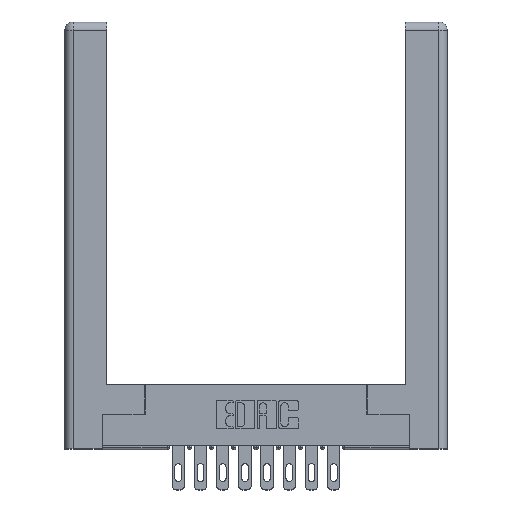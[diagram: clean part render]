
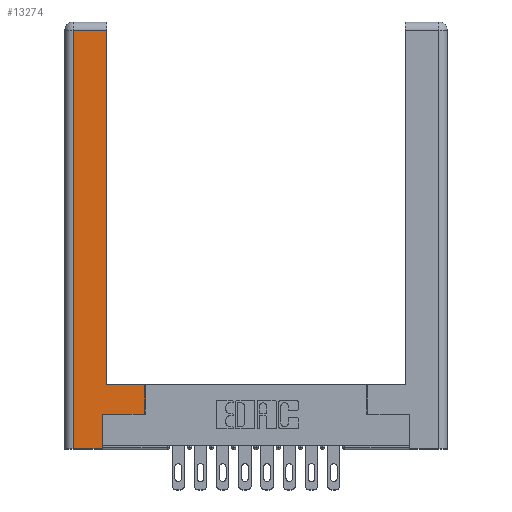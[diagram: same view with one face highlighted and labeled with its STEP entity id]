
A CAD part, top view. The second image highlights one B-rep face of the part: STEP entity #13274.
In plain terms, the highlighted planar face has unit normal (0, 0, 1).
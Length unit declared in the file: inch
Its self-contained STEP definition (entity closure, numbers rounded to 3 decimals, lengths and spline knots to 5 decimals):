
#339 = LINE ( 'NONE', #1525, #8223 ) ;
#506 = VECTOR ( 'NONE', #8954, 39.37008 ) ;
#558 = DIRECTION ( 'NONE',  ( 0., 1., 0. ) ) ;
#569 = VECTOR ( 'NONE', #4293, 39.37008 ) ;
#629 = AXIS2_PLACEMENT_3D ( 'NONE', #14079, #3267, #5479 ) ;
#686 = CARTESIAN_POINT ( 'NONE',  ( 0.265, 0.245, 0. ) ) ;
#910 = DIRECTION ( 'NONE',  ( 0., 1., 0. ) ) ;
#974 = VECTOR ( 'NONE', #3729, 39.37008 ) ;
#1103 = CARTESIAN_POINT ( 'NONE',  ( 0.0615, 2.94, 0. ) ) ;
#1105 = VECTOR ( 'NONE', #558, 39.37008 ) ;
#1204 = LINE ( 'NONE', #13820, #974 ) ;
#1525 = CARTESIAN_POINT ( 'NONE',  ( 0.0615, 0., 0. ) ) ;
#1530 = CARTESIAN_POINT ( 'NONE',  ( 0.565, 0.45, 0. ) ) ;
#2110 = CARTESIAN_POINT ( 'NONE',  ( 0.265, 0., 0. ) ) ;
#2571 = VERTEX_POINT ( 'NONE', #13230 ) ;
#2823 = LINE ( 'NONE', #7333, #4536 ) ;
#2871 = CARTESIAN_POINT ( 'NONE',  ( 0.265, 0.245, 0. ) ) ;
#3155 = LINE ( 'NONE', #12274, #4208 ) ;
#3267 = DIRECTION ( 'NONE',  ( 0., 0., -1. ) ) ;
#3407 = CARTESIAN_POINT ( 'NONE',  ( 0.0615, 2.94, 0. ) ) ;
#3729 = DIRECTION ( 'NONE',  ( 1., 0., 0. ) ) ;
#3953 = VERTEX_POINT ( 'NONE', #7651 ) ;
#4208 = VECTOR ( 'NONE', #910, 39.37008 ) ;
#4293 = DIRECTION ( 'NONE',  ( -1., 0., 0. ) ) ;
#4536 = VECTOR ( 'NONE', #11867, 39.37008 ) ;
#4557 = ORIENTED_EDGE ( 'NONE', *, *, #8539, .T. ) ;
#4577 = VECTOR ( 'NONE', #11735, 39.37008 ) ;
#4858 = DIRECTION ( 'NONE',  ( 0., -1., 0. ) ) ;
#5479 = DIRECTION ( 'NONE',  ( -1., 0., 0. ) ) ;
#5654 = ORIENTED_EDGE ( 'NONE', *, *, #13636, .T. ) ;
#5947 = LINE ( 'NONE', #11664, #4577 ) ;
#5993 = EDGE_CURVE ( 'NONE', #14133, #3953, #1204, .T. ) ;
#6494 = EDGE_CURVE ( 'NONE', #13491, #14245, #2823, .T. ) ;
#6582 = ORIENTED_EDGE ( 'NONE', *, *, #14240, .T. ) ;
#6707 = ORIENTED_EDGE ( 'NONE', *, *, #6781, .T. ) ;
#6781 = EDGE_CURVE ( 'NONE', #10850, #2571, #13476, .T. ) ;
#7333 = CARTESIAN_POINT ( 'NONE',  ( 0.265, 0., 0. ) ) ;
#7483 = ORIENTED_EDGE ( 'NONE', *, *, #5993, .T. ) ;
#7651 = CARTESIAN_POINT ( 'NONE',  ( 0.565, 0.245, 0. ) ) ;
#7898 = ORIENTED_EDGE ( 'NONE', *, *, #13544, .T. ) ;
#8223 = VECTOR ( 'NONE', #4858, 39.37008 ) ;
#8307 = ORIENTED_EDGE ( 'NONE', *, *, #11016, .T. ) ;
#8539 = EDGE_CURVE ( 'NONE', #9293, #10850, #5947, .T. ) ;
#8954 = DIRECTION ( 'NONE',  ( 0., 1., 0. ) ) ;
#9257 = CARTESIAN_POINT ( 'NONE',  ( 0.0615, 0., 0. ) ) ;
#9293 = VERTEX_POINT ( 'NONE', #1530 ) ;
#9565 = PLANE ( 'NONE',  #629 ) ;
#9724 = CARTESIAN_POINT ( 'NONE',  ( 0.295, 0.45, 0. ) ) ;
#10850 = VERTEX_POINT ( 'NONE', #9724 ) ;
#11016 = EDGE_CURVE ( 'NONE', #2571, #12965, #11210, .T. ) ;
#11028 = CARTESIAN_POINT ( 'NONE',  ( 0.295, 3., 0. ) ) ;
#11210 = LINE ( 'NONE', #3407, #569 ) ;
#11664 = CARTESIAN_POINT ( 'NONE',  ( 0.295, 0.45, 0. ) ) ;
#11735 = DIRECTION ( 'NONE',  ( -1., 0., 0. ) ) ;
#11842 = LINE ( 'NONE', #2871, #1105 ) ;
#11867 = DIRECTION ( 'NONE',  ( 1., 0., 0. ) ) ;
#12274 = CARTESIAN_POINT ( 'NONE',  ( 0.565, 0.45, 0. ) ) ;
#12542 = EDGE_LOOP ( 'NONE', ( #6707, #8307, #7898, #13065, #5654, #7483, #6582, #4557 ) ) ;
#12965 = VERTEX_POINT ( 'NONE', #1103 ) ;
#13065 = ORIENTED_EDGE ( 'NONE', *, *, #6494, .T. ) ;
#13230 = CARTESIAN_POINT ( 'NONE',  ( 0.295, 2.94, 0. ) ) ;
#13273 = FACE_OUTER_BOUND ( 'NONE', #12542, .T. ) ;
#13274 = ADVANCED_FACE ( 'NONE', ( #13273 ), #9565, .F. ) ;
#13476 = LINE ( 'NONE', #11028, #506 ) ;
#13491 = VERTEX_POINT ( 'NONE', #9257 ) ;
#13544 = EDGE_CURVE ( 'NONE', #12965, #13491, #339, .T. ) ;
#13636 = EDGE_CURVE ( 'NONE', #14245, #14133, #11842, .T. ) ;
#13820 = CARTESIAN_POINT ( 'NONE',  ( 0.565, 0.245, 0. ) ) ;
#14079 = CARTESIAN_POINT ( 'NONE',  ( 0., 0., 0. ) ) ;
#14133 = VERTEX_POINT ( 'NONE', #686 ) ;
#14240 = EDGE_CURVE ( 'NONE', #3953, #9293, #3155, .T. ) ;
#14245 = VERTEX_POINT ( 'NONE', #2110 ) ;
